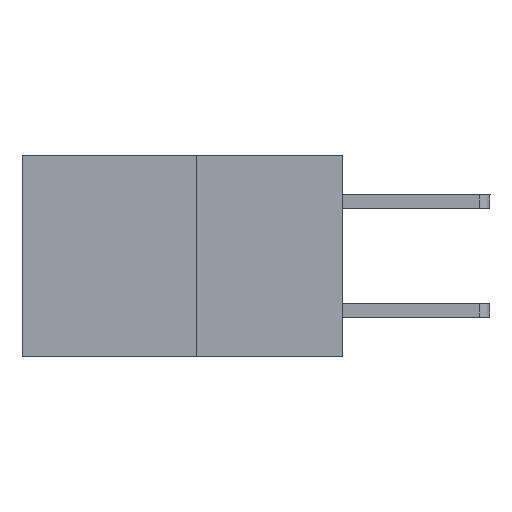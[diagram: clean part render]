
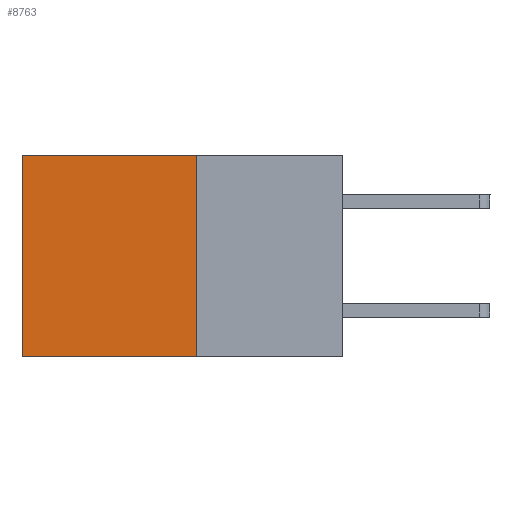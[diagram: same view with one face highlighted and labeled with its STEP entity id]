
A CAD part, left-side view. The second image highlights one B-rep face of the part: STEP entity #8763.
In plain terms, the highlighted planar face has unit normal (-1, 0, 0).
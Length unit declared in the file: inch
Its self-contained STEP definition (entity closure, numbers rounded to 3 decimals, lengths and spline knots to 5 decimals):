
#81 = EDGE_CURVE ( 'NONE', #8843, #1945, #3678, .T. ) ;
#159 = DIRECTION ( 'NONE',  ( 1., 0., 0. ) ) ;
#399 = CARTESIAN_POINT ( 'NONE',  ( 0.277, 0.59, 0. ) ) ;
#478 = DIRECTION ( 'NONE',  ( 0., 1., 0. ) ) ;
#509 = VERTEX_POINT ( 'NONE', #7162 ) ;
#989 = LINE ( 'NONE', #3871, #4133 ) ;
#1015 = DIRECTION ( 'NONE',  ( 0., 1., 0. ) ) ;
#1193 = LINE ( 'NONE', #4082, #7273 ) ;
#1429 = ORIENTED_EDGE ( 'NONE', *, *, #81, .T. ) ;
#1513 = ORIENTED_EDGE ( 'NONE', *, *, #3251, .F. ) ;
#1945 = VERTEX_POINT ( 'NONE', #2646 ) ;
#2126 = ORIENTED_EDGE ( 'NONE', *, *, #8129, .T. ) ;
#2257 = CARTESIAN_POINT ( 'NONE',  ( 0.277, 0.27, -0.37 ) ) ;
#2500 = CARTESIAN_POINT ( 'NONE',  ( 0.277, 0.27, -0.37 ) ) ;
#2646 = CARTESIAN_POINT ( 'NONE',  ( 0.277, 0.59, -0.37 ) ) ;
#3122 = DIRECTION ( 'NONE',  ( 0., 0., -1. ) ) ;
#3251 = EDGE_CURVE ( 'NONE', #6993, #509, #989, .T. ) ;
#3678 = LINE ( 'NONE', #7219, #6818 ) ;
#3871 = CARTESIAN_POINT ( 'NONE',  ( 0.277, 0.27, -0.37 ) ) ;
#4082 = CARTESIAN_POINT ( 'NONE',  ( 0.277, 0.27, 0. ) ) ;
#4133 = VECTOR ( 'NONE', #3122, 39.37008 ) ;
#4951 = VECTOR ( 'NONE', #1015, 39.37008 ) ;
#5843 = PLANE ( 'NONE',  #7720 ) ;
#6070 = CARTESIAN_POINT ( 'NONE',  ( 0.277, 0.27, 0. ) ) ;
#6645 = FACE_OUTER_BOUND ( 'NONE', #6838, .T. ) ;
#6701 = ORIENTED_EDGE ( 'NONE', *, *, #7043, .F. ) ;
#6818 = VECTOR ( 'NONE', #7262, 39.37008 ) ;
#6838 = EDGE_LOOP ( 'NONE', ( #1429, #6701, #1513, #2126 ) ) ;
#6993 = VERTEX_POINT ( 'NONE', #6070 ) ;
#7043 = EDGE_CURVE ( 'NONE', #509, #1945, #9115, .T. ) ;
#7162 = CARTESIAN_POINT ( 'NONE',  ( 0.277, 0.27, -0.37 ) ) ;
#7219 = CARTESIAN_POINT ( 'NONE',  ( 0.277, 0.59, -0.37 ) ) ;
#7262 = DIRECTION ( 'NONE',  ( 0., 0., -1. ) ) ;
#7273 = VECTOR ( 'NONE', #478, 39.37008 ) ;
#7405 = DIRECTION ( 'NONE',  ( 0., 0., -1. ) ) ;
#7720 = AXIS2_PLACEMENT_3D ( 'NONE', #2257, #159, #7405 ) ;
#8129 = EDGE_CURVE ( 'NONE', #6993, #8843, #1193, .T. ) ;
#8763 = ADVANCED_FACE ( 'NONE', ( #6645 ), #5843, .F. ) ;
#8843 = VERTEX_POINT ( 'NONE', #399 ) ;
#9115 = LINE ( 'NONE', #2500, #4951 ) ;
